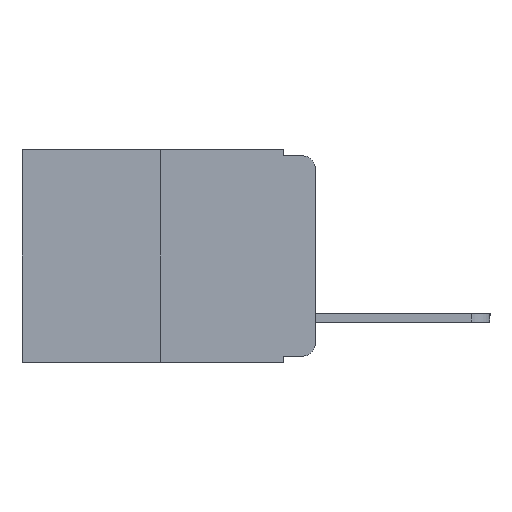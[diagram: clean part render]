
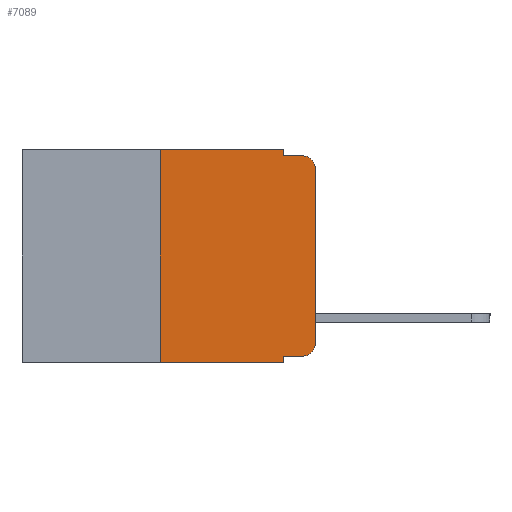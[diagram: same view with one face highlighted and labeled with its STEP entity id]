
A CAD part, left-side view. The second image highlights one B-rep face of the part: STEP entity #7089.
In plain terms, the highlighted planar face has unit normal (-1, 0, 0).
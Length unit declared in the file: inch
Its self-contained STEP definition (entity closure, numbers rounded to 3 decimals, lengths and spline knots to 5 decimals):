
#62 = CARTESIAN_POINT ( 'NONE',  ( 0., 0.051, 0. ) ) ;
#611 = VERTEX_POINT ( 'NONE', #9492 ) ;
#689 = VERTEX_POINT ( 'NONE', #9628 ) ;
#750 = CARTESIAN_POINT ( 'NONE',  ( 0., 0.25, 0. ) ) ;
#951 = DIRECTION ( 'NONE',  ( 0., 0., 1. ) ) ;
#1037 = LINE ( 'NONE', #9079, #1319 ) ;
#1204 = VERTEX_POINT ( 'NONE', #9802 ) ;
#1319 = VECTOR ( 'NONE', #9104, 39.37008 ) ;
#1371 = CARTESIAN_POINT ( 'NONE',  ( 0., 0.473, -0.343 ) ) ;
#1383 = DIRECTION ( 'NONE',  ( 0., -1., 0. ) ) ;
#1498 = CARTESIAN_POINT ( 'NONE',  ( 0., 0., 0. ) ) ;
#1694 = DIRECTION ( 'NONE',  ( -1., 0., 0. ) ) ;
#2259 = LINE ( 'NONE', #7148, #6333 ) ;
#2262 = EDGE_CURVE ( 'NONE', #4386, #3833, #6855, .T. ) ;
#2316 = ORIENTED_EDGE ( 'NONE', *, *, #3163, .T. ) ;
#2336 = EDGE_LOOP ( 'NONE', ( #2316, #2416, #2489, #2704, #2803, #2920, #3186, #3859, #4142, #4402 ) ) ;
#2416 = ORIENTED_EDGE ( 'NONE', *, *, #4552, .T. ) ;
#2456 = DIRECTION ( 'NONE',  ( 0., -1., 0. ) ) ;
#2489 = ORIENTED_EDGE ( 'NONE', *, *, #6590, .F. ) ;
#2704 = ORIENTED_EDGE ( 'NONE', *, *, #7047, .F. ) ;
#2707 = CARTESIAN_POINT ( 'NONE',  ( 0., 0.051, 0. ) ) ;
#2803 = ORIENTED_EDGE ( 'NONE', *, *, #4721, .F. ) ;
#2808 = VERTEX_POINT ( 'NONE', #10122 ) ;
#2920 = ORIENTED_EDGE ( 'NONE', *, *, #2262, .F. ) ;
#3163 = EDGE_CURVE ( 'NONE', #4676, #2808, #9750, .T. ) ;
#3178 = EDGE_CURVE ( 'NONE', #689, #611, #3688, .T. ) ;
#3186 = ORIENTED_EDGE ( 'NONE', *, *, #9484, .T. ) ;
#3440 = VECTOR ( 'NONE', #1383, 39.37008 ) ;
#3688 = LINE ( 'NONE', #62, #5610 ) ;
#3833 = VERTEX_POINT ( 'NONE', #6348 ) ;
#3859 = ORIENTED_EDGE ( 'NONE', *, *, #3178, .F. ) ;
#3887 = DIRECTION ( 'NONE',  ( 0., 0., 1. ) ) ;
#4142 = ORIENTED_EDGE ( 'NONE', *, *, #5423, .T. ) ;
#4386 = VERTEX_POINT ( 'NONE', #6752 ) ;
#4402 = ORIENTED_EDGE ( 'NONE', *, *, #5921, .T. ) ;
#4552 = EDGE_CURVE ( 'NONE', #2808, #1204, #4838, .T. ) ;
#4554 = CARTESIAN_POINT ( 'NONE',  ( 0., 0.02, -0.313 ) ) ;
#4676 = VERTEX_POINT ( 'NONE', #6869 ) ;
#4721 = EDGE_CURVE ( 'NONE', #3833, #9212, #5453, .T. ) ;
#4838 = CIRCLE ( 'NONE', #6585, 0.02 ) ;
#5075 = VERTEX_POINT ( 'NONE', #7139 ) ;
#5190 = VECTOR ( 'NONE', #6699, 39.37008 ) ;
#5423 = EDGE_CURVE ( 'NONE', #689, #5075, #8364, .T. ) ;
#5453 = LINE ( 'NONE', #6537, #5190 ) ;
#5610 = VECTOR ( 'NONE', #9803, 39.37008 ) ;
#5702 = CARTESIAN_POINT ( 'NONE',  ( 0., 0.051, -0.01 ) ) ;
#5780 = DIRECTION ( 'NONE',  ( 0., -1., 0. ) ) ;
#5810 = CARTESIAN_POINT ( 'NONE',  ( 0., 0.051, -0.333 ) ) ;
#5921 = EDGE_CURVE ( 'NONE', #5075, #4676, #6136, .T. ) ;
#5977 = DIRECTION ( 'NONE',  ( 0., 0., -1. ) ) ;
#6016 = DIRECTION ( 'NONE',  ( -1., 0., 0. ) ) ;
#6026 = CARTESIAN_POINT ( 'NONE',  ( 0., 0.02, -0.03 ) ) ;
#6136 = CIRCLE ( 'NONE', #10045, 0.02 ) ;
#6333 = VECTOR ( 'NONE', #5780, 39.37008 ) ;
#6348 = CARTESIAN_POINT ( 'NONE',  ( 0., 0.25, 0. ) ) ;
#6537 = CARTESIAN_POINT ( 'NONE',  ( 0., 0.473, 0. ) ) ;
#6583 = VECTOR ( 'NONE', #2456, 39.37008 ) ;
#6585 = AXIS2_PLACEMENT_3D ( 'NONE', #6026, #6016, #5977 ) ;
#6590 = EDGE_CURVE ( 'NONE', #9822, #1204, #2259, .T. ) ;
#6699 = DIRECTION ( 'NONE',  ( 0., -1., 0. ) ) ;
#6752 = CARTESIAN_POINT ( 'NONE',  ( 0., 0.25, -0.343 ) ) ;
#6855 = LINE ( 'NONE', #750, #8401 ) ;
#6869 = CARTESIAN_POINT ( 'NONE',  ( 0., 0., -0.313 ) ) ;
#7047 = EDGE_CURVE ( 'NONE', #9212, #9822, #1037, .T. ) ;
#7089 = ADVANCED_FACE ( 'NONE', ( #7215 ), #8755, .F. ) ;
#7139 = CARTESIAN_POINT ( 'NONE',  ( 0., 0.02, -0.333 ) ) ;
#7148 = CARTESIAN_POINT ( 'NONE',  ( 0., 0.051, -0.01 ) ) ;
#7215 = FACE_OUTER_BOUND ( 'NONE', #2336, .T. ) ;
#7468 = DIRECTION ( 'NONE',  ( 0., 0., -1. ) ) ;
#7666 = VECTOR ( 'NONE', #3887, 39.37008 ) ;
#8364 = LINE ( 'NONE', #5810, #6583 ) ;
#8401 = VECTOR ( 'NONE', #951, 39.37008 ) ;
#8649 = AXIS2_PLACEMENT_3D ( 'NONE', #8887, #8882, #8857 ) ;
#8755 = PLANE ( 'NONE',  #8649 ) ;
#8857 = DIRECTION ( 'NONE',  ( 0., 0., -1. ) ) ;
#8872 = LINE ( 'NONE', #1371, #3440 ) ;
#8882 = DIRECTION ( 'NONE',  ( 1., 0., 0. ) ) ;
#8887 = CARTESIAN_POINT ( 'NONE',  ( 0., 0.473, 0. ) ) ;
#9079 = CARTESIAN_POINT ( 'NONE',  ( 0., 0.051, 0. ) ) ;
#9104 = DIRECTION ( 'NONE',  ( 0., 0., -1. ) ) ;
#9212 = VERTEX_POINT ( 'NONE', #2707 ) ;
#9484 = EDGE_CURVE ( 'NONE', #4386, #611, #8872, .T. ) ;
#9492 = CARTESIAN_POINT ( 'NONE',  ( 0., 0.051, -0.343 ) ) ;
#9628 = CARTESIAN_POINT ( 'NONE',  ( 0., 0.051, -0.333 ) ) ;
#9750 = LINE ( 'NONE', #1498, #7666 ) ;
#9802 = CARTESIAN_POINT ( 'NONE',  ( 0., 0.02, -0.01 ) ) ;
#9803 = DIRECTION ( 'NONE',  ( 0., 0., -1. ) ) ;
#9822 = VERTEX_POINT ( 'NONE', #5702 ) ;
#10045 = AXIS2_PLACEMENT_3D ( 'NONE', #4554, #1694, #7468 ) ;
#10122 = CARTESIAN_POINT ( 'NONE',  ( 0., 0., -0.03 ) ) ;
